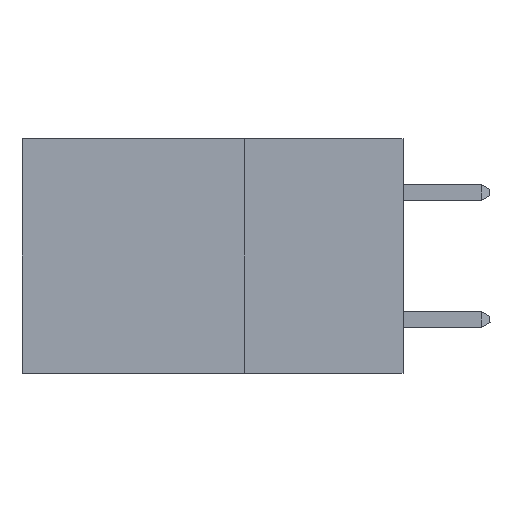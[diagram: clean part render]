
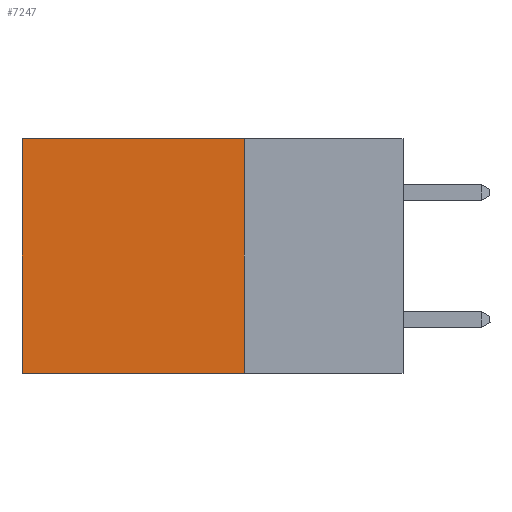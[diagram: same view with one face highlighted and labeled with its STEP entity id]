
A CAD part, left-side view. The second image highlights one B-rep face of the part: STEP entity #7247.
In plain terms, the highlighted planar face has unit normal (-1, 0, 0).
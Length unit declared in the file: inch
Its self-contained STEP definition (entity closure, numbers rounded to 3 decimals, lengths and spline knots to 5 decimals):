
#584 = VERTEX_POINT ( 'NONE', #13789 ) ;
#1231 = DIRECTION ( 'NONE',  ( 0., 1., 0. ) ) ;
#1543 = EDGE_CURVE ( 'NONE', #28400, #19275, #26018, .T. ) ;
#4597 = AXIS2_PLACEMENT_3D ( 'NONE', #17199, #29205, #11738 ) ;
#6010 = PLANE ( 'NONE',  #4597 ) ;
#7247 = ADVANCED_FACE ( 'NONE', ( #19186 ), #6010, .F. ) ;
#7374 = DIRECTION ( 'NONE',  ( 0., 0., -1. ) ) ;
#7469 = CARTESIAN_POINT ( 'NONE',  ( 0.2875, 0.25, -0.37 ) ) ;
#8116 = EDGE_LOOP ( 'NONE', ( #14000, #29828, #13538, #29985 ) ) ;
#8508 = CARTESIAN_POINT ( 'NONE',  ( 0.2875, 0.6, 0. ) ) ;
#10462 = LINE ( 'NONE', #25063, #24536 ) ;
#10661 = VECTOR ( 'NONE', #23003, 39.37008 ) ;
#11738 = DIRECTION ( 'NONE',  ( 0., 0., -1. ) ) ;
#13538 = ORIENTED_EDGE ( 'NONE', *, *, #1543, .F. ) ;
#13789 = CARTESIAN_POINT ( 'NONE',  ( 0.2875, 0.6, -0.37 ) ) ;
#14000 = ORIENTED_EDGE ( 'NONE', *, *, #31120, .T. ) ;
#14444 = LINE ( 'NONE', #7469, #37521 ) ;
#17199 = CARTESIAN_POINT ( 'NONE',  ( 0.2875, 0.25, 0. ) ) ;
#19186 = FACE_OUTER_BOUND ( 'NONE', #8116, .T. ) ;
#19200 = DIRECTION ( 'NONE',  ( 0., 1., 0. ) ) ;
#19275 = VERTEX_POINT ( 'NONE', #28625 ) ;
#21817 = CARTESIAN_POINT ( 'NONE',  ( 0.2875, 0.25, 0. ) ) ;
#22366 = CARTESIAN_POINT ( 'NONE',  ( 0.2875, 0.25, 0. ) ) ;
#23003 = DIRECTION ( 'NONE',  ( 0., 0., -1. ) ) ;
#23284 = CARTESIAN_POINT ( 'NONE',  ( 0.2875, 0.6, 0. ) ) ;
#24536 = VECTOR ( 'NONE', #19200, 39.37008 ) ;
#25063 = CARTESIAN_POINT ( 'NONE',  ( 0.2875, 0.25, 0. ) ) ;
#26018 = LINE ( 'NONE', #21817, #30534 ) ;
#28400 = VERTEX_POINT ( 'NONE', #22366 ) ;
#28625 = CARTESIAN_POINT ( 'NONE',  ( 0.2875, 0.25, -0.37 ) ) ;
#29205 = DIRECTION ( 'NONE',  ( 1., 0., 0. ) ) ;
#29828 = ORIENTED_EDGE ( 'NONE', *, *, #35799, .F. ) ;
#29985 = ORIENTED_EDGE ( 'NONE', *, *, #34044, .T. ) ;
#30534 = VECTOR ( 'NONE', #7374, 39.37008 ) ;
#30546 = VERTEX_POINT ( 'NONE', #23284 ) ;
#31120 = EDGE_CURVE ( 'NONE', #30546, #584, #32353, .T. ) ;
#32353 = LINE ( 'NONE', #8508, #10661 ) ;
#34044 = EDGE_CURVE ( 'NONE', #28400, #30546, #10462, .T. ) ;
#35799 = EDGE_CURVE ( 'NONE', #19275, #584, #14444, .T. ) ;
#37521 = VECTOR ( 'NONE', #1231, 39.37008 ) ;
